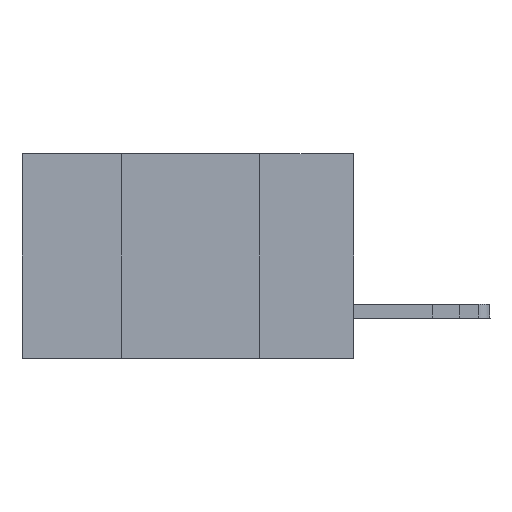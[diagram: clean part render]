
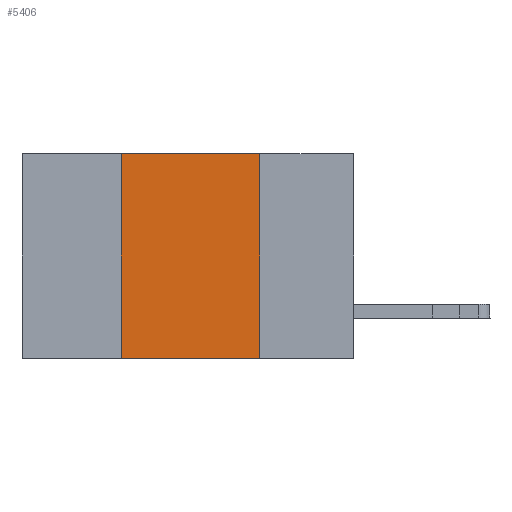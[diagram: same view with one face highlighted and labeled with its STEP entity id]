
A CAD part, left-side view. The second image highlights one B-rep face of the part: STEP entity #5406.
In plain terms, the highlighted planar face has unit normal (-1, 0, 0).
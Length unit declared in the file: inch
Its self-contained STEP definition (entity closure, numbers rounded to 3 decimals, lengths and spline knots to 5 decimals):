
#1387 = DIRECTION ( 'NONE',  ( 0., 0., -1. ) ) ;
#1757 = AXIS2_PLACEMENT_3D ( 'NONE', #3143, #15505, #1387 ) ;
#1787 = CARTESIAN_POINT ( 'NONE',  ( 0., 0.6, 0. ) ) ;
#1986 = CARTESIAN_POINT ( 'NONE',  ( 0., 0.42, 0. ) ) ;
#3143 = CARTESIAN_POINT ( 'NONE',  ( 0., 0.6, 0. ) ) ;
#5406 = ADVANCED_FACE ( 'NONE', ( #6758 ), #12044, .F. ) ;
#5642 = ORIENTED_EDGE ( 'NONE', *, *, #21247, .F. ) ;
#5889 = ORIENTED_EDGE ( 'NONE', *, *, #18608, .F. ) ;
#6069 = DIRECTION ( 'NONE',  ( 0., 0., -1. ) ) ;
#6758 = FACE_OUTER_BOUND ( 'NONE', #17936, .T. ) ;
#8315 = CARTESIAN_POINT ( 'NONE',  ( 0., 0.42, 0. ) ) ;
#8798 = LINE ( 'NONE', #14059, #22437 ) ;
#9038 = EDGE_CURVE ( 'NONE', #20845, #13245, #17756, .T. ) ;
#10878 = VECTOR ( 'NONE', #12755, 39.37008 ) ;
#11488 = CARTESIAN_POINT ( 'NONE',  ( 0., 0.17, 0. ) ) ;
#12044 = PLANE ( 'NONE',  #1757 ) ;
#12192 = DIRECTION ( 'NONE',  ( 0., -1., 0. ) ) ;
#12755 = DIRECTION ( 'NONE',  ( 0., 0., 1. ) ) ;
#12759 = VECTOR ( 'NONE', #6069, 39.37008 ) ;
#13245 = VERTEX_POINT ( 'NONE', #19959 ) ;
#14059 = CARTESIAN_POINT ( 'NONE',  ( 0., 0.6, -0.37 ) ) ;
#14235 = ORIENTED_EDGE ( 'NONE', *, *, #9038, .F. ) ;
#14739 = CARTESIAN_POINT ( 'NONE',  ( 0., 0.17, -0.37 ) ) ;
#15505 = DIRECTION ( 'NONE',  ( 1., 0., 0. ) ) ;
#17251 = LINE ( 'NONE', #11488, #12759 ) ;
#17756 = LINE ( 'NONE', #1787, #22694 ) ;
#17936 = EDGE_LOOP ( 'NONE', ( #5889, #14235, #5642, #21811 ) ) ;
#18608 = EDGE_CURVE ( 'NONE', #13245, #22308, #17251, .T. ) ;
#19384 = DIRECTION ( 'NONE',  ( 0., -1., 0. ) ) ;
#19583 = EDGE_CURVE ( 'NONE', #19740, #22308, #8798, .T. ) ;
#19703 = LINE ( 'NONE', #1986, #10878 ) ;
#19740 = VERTEX_POINT ( 'NONE', #19964 ) ;
#19959 = CARTESIAN_POINT ( 'NONE',  ( 0., 0.17, 0. ) ) ;
#19964 = CARTESIAN_POINT ( 'NONE',  ( 0., 0.42, -0.37 ) ) ;
#20845 = VERTEX_POINT ( 'NONE', #8315 ) ;
#21247 = EDGE_CURVE ( 'NONE', #19740, #20845, #19703, .T. ) ;
#21811 = ORIENTED_EDGE ( 'NONE', *, *, #19583, .T. ) ;
#22308 = VERTEX_POINT ( 'NONE', #14739 ) ;
#22437 = VECTOR ( 'NONE', #12192, 39.37008 ) ;
#22694 = VECTOR ( 'NONE', #19384, 39.37008 ) ;
